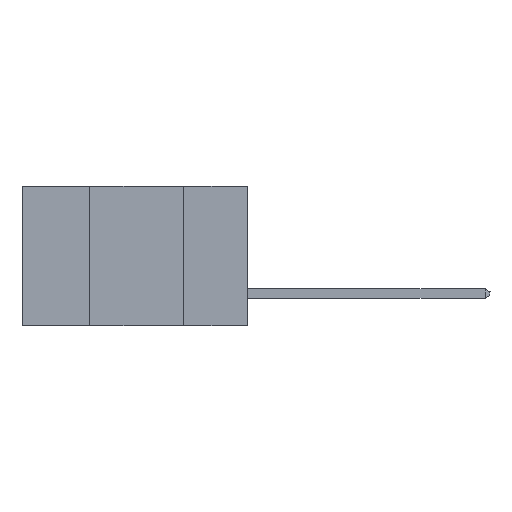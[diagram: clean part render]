
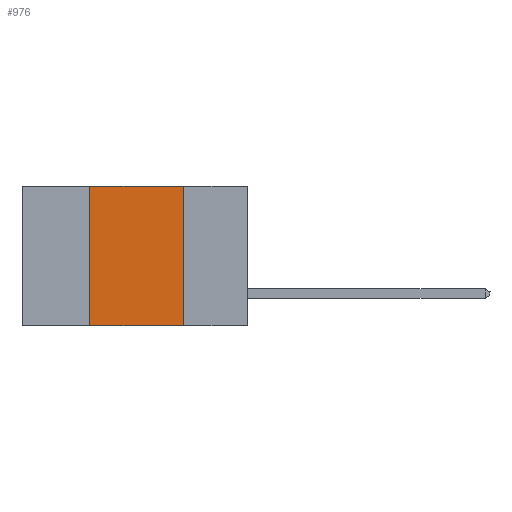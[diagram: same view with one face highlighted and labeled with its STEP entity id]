
A CAD part, left-side view. The second image highlights one B-rep face of the part: STEP entity #976.
In plain terms, the highlighted planar face has unit normal (-1, 0, 0).
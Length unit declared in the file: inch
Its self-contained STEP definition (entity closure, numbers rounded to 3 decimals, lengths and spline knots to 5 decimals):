
#238 = VECTOR ( 'NONE', #6297, 39.37008 ) ;
#338 = ORIENTED_EDGE ( 'NONE', *, *, #4730, .F. ) ;
#541 = VERTEX_POINT ( 'NONE', #11094 ) ;
#610 = VERTEX_POINT ( 'NONE', #2439 ) ;
#835 = FACE_OUTER_BOUND ( 'NONE', #4570, .T. ) ;
#863 = LINE ( 'NONE', #8876, #12128 ) ;
#976 = ADVANCED_FACE ( 'NONE', ( #835 ), #3636, .F. ) ;
#1676 = AXIS2_PLACEMENT_3D ( 'NONE', #5505, #11355, #3760 ) ;
#1685 = ORIENTED_EDGE ( 'NONE', *, *, #7317, .F. ) ;
#1729 = VERTEX_POINT ( 'NONE', #3267 ) ;
#1978 = CARTESIAN_POINT ( 'NONE',  ( 0., 0.6, -0.37 ) ) ;
#2439 = CARTESIAN_POINT ( 'NONE',  ( 0., 0.42, 0. ) ) ;
#2676 = ORIENTED_EDGE ( 'NONE', *, *, #11111, .F. ) ;
#3267 = CARTESIAN_POINT ( 'NONE',  ( 0., 0.42, -0.37 ) ) ;
#3426 = VERTEX_POINT ( 'NONE', #9733 ) ;
#3636 = PLANE ( 'NONE',  #1676 ) ;
#3760 = DIRECTION ( 'NONE',  ( 0., 0., -1. ) ) ;
#4570 = EDGE_LOOP ( 'NONE', ( #2676, #1685, #338, #5620 ) ) ;
#4730 = EDGE_CURVE ( 'NONE', #1729, #610, #5242, .T. ) ;
#4780 = LINE ( 'NONE', #5689, #12052 ) ;
#5242 = LINE ( 'NONE', #8150, #238 ) ;
#5505 = CARTESIAN_POINT ( 'NONE',  ( 0., 0.6, 0. ) ) ;
#5620 = ORIENTED_EDGE ( 'NONE', *, *, #10283, .T. ) ;
#5689 = CARTESIAN_POINT ( 'NONE',  ( 0., 0.6, 0. ) ) ;
#5809 = LINE ( 'NONE', #1978, #12315 ) ;
#6297 = DIRECTION ( 'NONE',  ( 0., 0., 1. ) ) ;
#6569 = DIRECTION ( 'NONE',  ( 0., -1., 0. ) ) ;
#7317 = EDGE_CURVE ( 'NONE', #610, #3426, #4780, .T. ) ;
#8150 = CARTESIAN_POINT ( 'NONE',  ( 0., 0.42, -0.37 ) ) ;
#8810 = DIRECTION ( 'NONE',  ( 0., 0., -1. ) ) ;
#8876 = CARTESIAN_POINT ( 'NONE',  ( 0., 0.17, -0.37 ) ) ;
#9681 = DIRECTION ( 'NONE',  ( 0., -1., 0. ) ) ;
#9733 = CARTESIAN_POINT ( 'NONE',  ( 0., 0.17, 0. ) ) ;
#10283 = EDGE_CURVE ( 'NONE', #1729, #541, #5809, .T. ) ;
#11094 = CARTESIAN_POINT ( 'NONE',  ( 0., 0.17, -0.37 ) ) ;
#11111 = EDGE_CURVE ( 'NONE', #3426, #541, #863, .T. ) ;
#11355 = DIRECTION ( 'NONE',  ( 1., 0., 0. ) ) ;
#12052 = VECTOR ( 'NONE', #6569, 39.37008 ) ;
#12128 = VECTOR ( 'NONE', #8810, 39.37008 ) ;
#12315 = VECTOR ( 'NONE', #9681, 39.37008 ) ;
